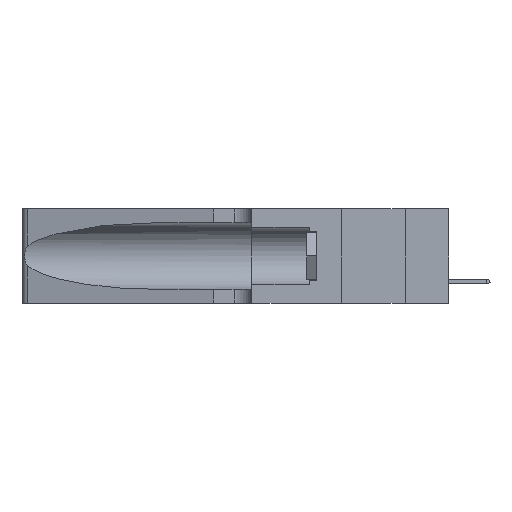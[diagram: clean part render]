
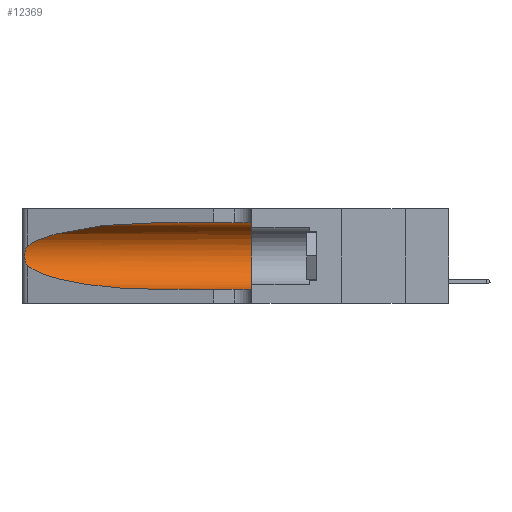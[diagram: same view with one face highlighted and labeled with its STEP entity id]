
A CAD part, left-side view. The second image highlights one B-rep face of the part: STEP entity #12369.
In plain terms, the highlighted cylindrical face has radius 3.308 mm (diameter 6.617 mm), a partial arc.
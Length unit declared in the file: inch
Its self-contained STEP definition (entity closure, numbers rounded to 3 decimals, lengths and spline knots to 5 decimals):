
#13 = CARTESIAN_POINT ( 'NONE',  ( 0.25639, 1.23184, 0.21858 ) ) ;
#184 = CARTESIAN_POINT ( 'NONE',  ( 0.1305, 0.72297, 0.31525 ) ) ;
#322 = B_SPLINE_CURVE_WITH_KNOTS ( 'NONE', 3,
 ( #7384, #7452, #13, #17519, #13120, #2727, #14785, #10403, #5768, #8819, #5969, #14665, #16279, #8882 ),
 .UNSPECIFIED., .F., .F.,
 ( 4, 2, 2, 2, 2, 2, 4 ),
 ( 0., 0.00027, 0.00053, 0.00107, 0.0016, 0.00187, 0.00214 ),
 .UNSPECIFIED. ) ;
#394 = DIRECTION ( 'NONE',  ( 0., -1., 0. ) ) ;
#1479 = CARTESIAN_POINT ( 'NONE',  ( 0.18966, 0.96281, 0.05475 ) ) ;
#2256 = ORIENTED_EDGE ( 'NONE', *, *, #2478, .T. ) ;
#2322 = ORIENTED_EDGE ( 'NONE', *, *, #11406, .F. ) ;
#2426 = LINE ( 'NONE', #16582, #9359 ) ;
#2478 = EDGE_CURVE ( 'NONE', #17036, #10731, #4935, .T. ) ;
#2715 = CARTESIAN_POINT ( 'NONE',  ( 0.25487, 1.22718, 0.22369 ) ) ;
#2727 = CARTESIAN_POINT ( 'NONE',  ( 0.26018, 1.23835, 0.19895 ) ) ;
#2993 = EDGE_LOOP ( 'NONE', ( #7230, #15032, #2256, #11322, #2322, #5471 ) ) ;
#3314 = AXIS2_PLACEMENT_3D ( 'NONE', #12393, #394, #4843 ) ;
#4843 = DIRECTION ( 'NONE',  ( 0., 0., -1. ) ) ;
#4935 =( BOUNDED_CURVE ( )  B_SPLINE_CURVE ( 3, ( #17755, #10210, #1479, #16265 ),
 .UNSPECIFIED., .F., .T. ) 
 B_SPLINE_CURVE_WITH_KNOTS ( ( 4, 4 ),
 ( 3.44316, 4.71239 ),
 .UNSPECIFIED. ) 
 CURVE ( )  GEOMETRIC_REPRESENTATION_ITEM ( )  RATIONAL_B_SPLINE_CURVE ( ( 1., 0.87, 0.87, 1. ) ) 
 REPRESENTATION_ITEM ( '' )  );
#5062 = DIRECTION ( 'NONE',  ( 0., 0., 1. ) ) ;
#5471 = ORIENTED_EDGE ( 'NONE', *, *, #12836, .F. ) ;
#5768 = CARTESIAN_POINT ( 'NONE',  ( 0.26017, 1.23833, 0.17102 ) ) ;
#5792 = AXIS2_PLACEMENT_3D ( 'NONE', #12203, #16352, #5062 ) ;
#5969 = CARTESIAN_POINT ( 'NONE',  ( 0.25789, 1.23486, 0.15765 ) ) ;
#6406 = DIRECTION ( 'NONE',  ( 0., -1., 0. ) ) ;
#6580 = VERTEX_POINT ( 'NONE', #7628 ) ;
#6622 = VECTOR ( 'NONE', #15422, 39.37008 ) ;
#7230 = ORIENTED_EDGE ( 'NONE', *, *, #7650, .T. ) ;
#7384 = CARTESIAN_POINT ( 'NONE',  ( 0.25487, 1.22718, 0.22369 ) ) ;
#7452 = CARTESIAN_POINT ( 'NONE',  ( 0.25555, 1.22994, 0.2215 ) ) ;
#7628 = CARTESIAN_POINT ( 'NONE',  ( 0.1305, 0.35, 0.31525 ) ) ;
#7650 = EDGE_CURVE ( 'NONE', #17073, #8050, #9209, .T. ) ;
#8050 = VERTEX_POINT ( 'NONE', #2715 ) ;
#8819 = CARTESIAN_POINT ( 'NONE',  ( 0.25856, 1.23593, 0.16098 ) ) ;
#8882 = CARTESIAN_POINT ( 'NONE',  ( 0.25487, 1.22718, 0.14631 ) ) ;
#9209 =( BOUNDED_CURVE ( )  B_SPLINE_CURVE ( 3, ( #184, #16391, #16326, #11857 ),
 .UNSPECIFIED., .F., .T. ) 
 B_SPLINE_CURVE_WITH_KNOTS ( ( 4, 4 ),
 ( 1.5708, 2.84003 ),
 .UNSPECIFIED. ) 
 CURVE ( )  GEOMETRIC_REPRESENTATION_ITEM ( )  RATIONAL_B_SPLINE_CURVE ( ( 1., 0.87, 0.87, 1. ) ) 
 REPRESENTATION_ITEM ( '' )  );
#9297 = CARTESIAN_POINT ( 'NONE',  ( 0.1305, 1.61858, 0.05475 ) ) ;
#9359 = VECTOR ( 'NONE', #6406, 39.37008 ) ;
#10071 = FACE_OUTER_BOUND ( 'NONE', #2993, .T. ) ;
#10210 = CARTESIAN_POINT ( 'NONE',  ( 0.2373, 1.15595, 0.08982 ) ) ;
#10403 = CARTESIAN_POINT ( 'NONE',  ( 0.26075, 1.23896, 0.178 ) ) ;
#10731 = VERTEX_POINT ( 'NONE', #15282 ) ;
#11322 = ORIENTED_EDGE ( 'NONE', *, *, #14035, .T. ) ;
#11393 = VERTEX_POINT ( 'NONE', #15007 ) ;
#11406 = EDGE_CURVE ( 'NONE', #6580, #11393, #18413, .T. ) ;
#11857 = CARTESIAN_POINT ( 'NONE',  ( 0.25487, 1.22718, 0.22369 ) ) ;
#12203 = CARTESIAN_POINT ( 'NONE',  ( 0.1305, 0.35, 0.185 ) ) ;
#12369 = ADVANCED_FACE ( 'NONE', ( #10071 ), #16518, .F. ) ;
#12393 = CARTESIAN_POINT ( 'NONE',  ( 0.1305, 1.61858, 0.185 ) ) ;
#12836 = EDGE_CURVE ( 'NONE', #17073, #6580, #2426, .T. ) ;
#13120 = CARTESIAN_POINT ( 'NONE',  ( 0.25854, 1.2359, 0.20912 ) ) ;
#13522 = LINE ( 'NONE', #9297, #6622 ) ;
#14035 = EDGE_CURVE ( 'NONE', #10731, #11393, #13522, .T. ) ;
#14665 = CARTESIAN_POINT ( 'NONE',  ( 0.25639, 1.23186, 0.15144 ) ) ;
#14785 = CARTESIAN_POINT ( 'NONE',  ( 0.26075, 1.23896, 0.19203 ) ) ;
#15007 = CARTESIAN_POINT ( 'NONE',  ( 0.1305, 0.35, 0.05475 ) ) ;
#15032 = ORIENTED_EDGE ( 'NONE', *, *, #18240, .T. ) ;
#15282 = CARTESIAN_POINT ( 'NONE',  ( 0.1305, 0.72297, 0.05475 ) ) ;
#15422 = DIRECTION ( 'NONE',  ( 0., -1., 0. ) ) ;
#16265 = CARTESIAN_POINT ( 'NONE',  ( 0.1305, 0.72297, 0.05475 ) ) ;
#16279 = CARTESIAN_POINT ( 'NONE',  ( 0.25555, 1.22993, 0.14849 ) ) ;
#16326 = CARTESIAN_POINT ( 'NONE',  ( 0.2373, 1.15595, 0.28018 ) ) ;
#16352 = DIRECTION ( 'NONE',  ( 0., 1., 0. ) ) ;
#16391 = CARTESIAN_POINT ( 'NONE',  ( 0.18966, 0.96281, 0.31525 ) ) ;
#16518 = CYLINDRICAL_SURFACE ( 'NONE', #3314, 0.13025 ) ;
#16582 = CARTESIAN_POINT ( 'NONE',  ( 0.1305, 1.61858, 0.31525 ) ) ;
#17036 = VERTEX_POINT ( 'NONE', #17056 ) ;
#17056 = CARTESIAN_POINT ( 'NONE',  ( 0.25487, 1.22718, 0.14631 ) ) ;
#17073 = VERTEX_POINT ( 'NONE', #17116 ) ;
#17116 = CARTESIAN_POINT ( 'NONE',  ( 0.1305, 0.72297, 0.31525 ) ) ;
#17519 = CARTESIAN_POINT ( 'NONE',  ( 0.25787, 1.23484, 0.2124 ) ) ;
#17755 = CARTESIAN_POINT ( 'NONE',  ( 0.25487, 1.22718, 0.14631 ) ) ;
#18240 = EDGE_CURVE ( 'NONE', #8050, #17036, #322, .T. ) ;
#18413 = CIRCLE ( 'NONE', #5792, 0.13025 ) ;
